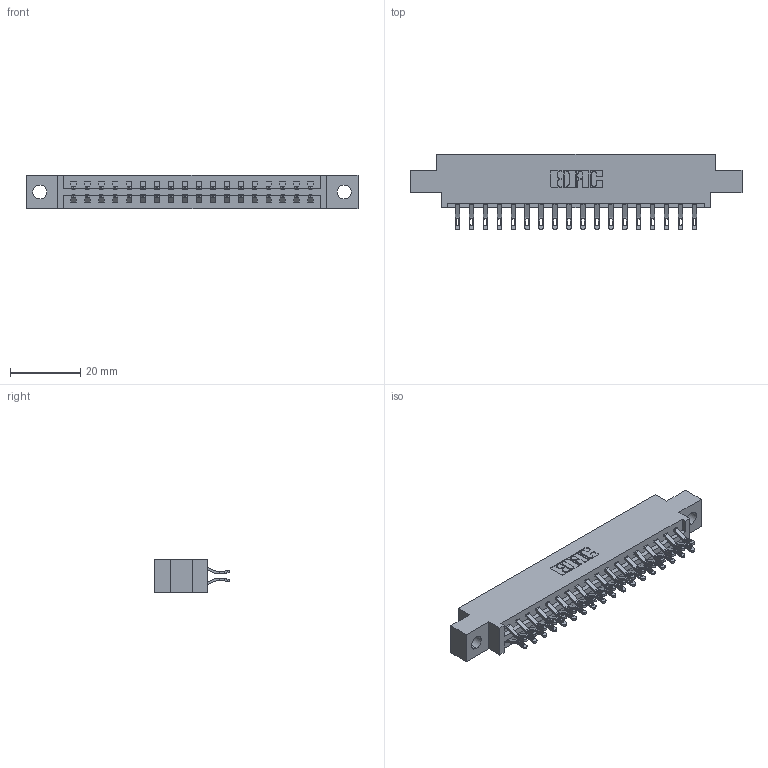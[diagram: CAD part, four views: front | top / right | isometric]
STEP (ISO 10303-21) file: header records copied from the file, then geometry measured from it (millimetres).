
FILE_DESCRIPTION (( 'STEP AP203' ), '1' );
FILE_NAME ('387-036-555-804.STEP', '2019-10-17T19:55:08', ( '' ), ( '' ), 'SwSTEP 2.0', 'SolidWorks 2016', '' );
FILE_SCHEMA (( 'CONFIG_CONTROL_DESIGN' ));
Length unit declared in the file: inch
Products named in the file (3): 387-036-555-804; 337 Part_0.170 Offset - 0.156 Dia-TH; 345-292-001_555 Tail
Assembly tree (37 placements, depth 2):
  387-036-555-804
    337 Part_0.170 Offset - 0.156 Dia-TH
    345-292-001_555 Tail  x36
Bounding box: 94.34 x 21.47 x 9.4 mm (x, y, z)
Volume: 9521.4 mm3; surface area: 10829.6 mm2
Topology: 37 solids, 37 shells, 2278 faces, 7127 edges, 4750 vertices
Faces by surface type: plane 1370, cylinder 908
Entity records: 17521 total; most frequent: CARTESIAN_POINT 3008, ORIENTED_EDGE 2914, DIRECTION 2573, EDGE_CURVE 1457, LINE 1309, VECTOR 1309, VERTEX_POINT 970, AXIS2_PLACEMENT_3D 632
